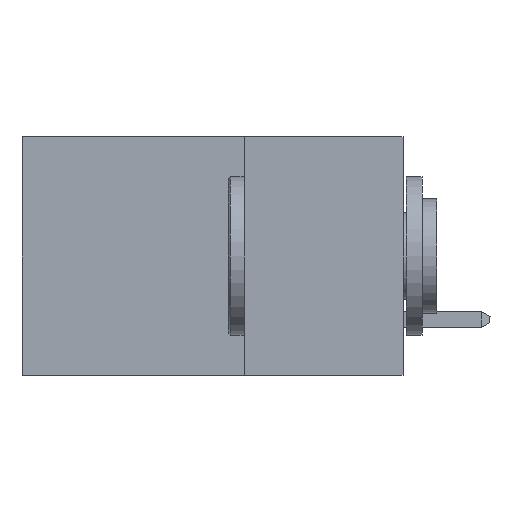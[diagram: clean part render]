
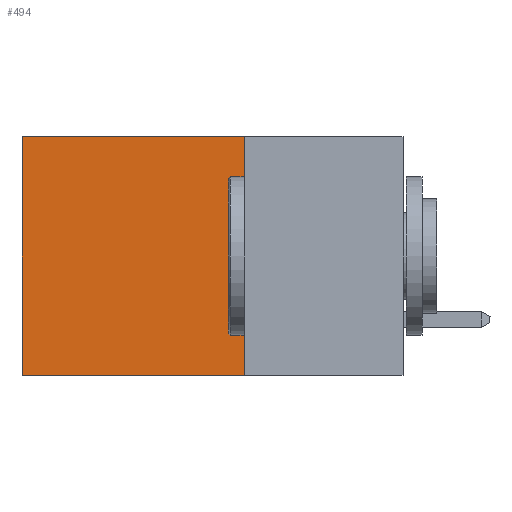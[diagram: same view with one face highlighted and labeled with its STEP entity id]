
A CAD part, left-side view. The second image highlights one B-rep face of the part: STEP entity #494.
In plain terms, the highlighted planar face has unit normal (-1, 0, 0).
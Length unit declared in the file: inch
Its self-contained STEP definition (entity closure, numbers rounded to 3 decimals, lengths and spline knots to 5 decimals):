
#149 = DIRECTION ( 'NONE',  ( 0., 0., -1. ) ) ;
#494 = ADVANCED_FACE ( 'NONE', ( #10853 ), #8749, .F. ) ;
#1987 = VECTOR ( 'NONE', #149, 39.37008 ) ;
#2050 = CARTESIAN_POINT ( 'NONE',  ( 0.2875, 0.25, 0. ) ) ;
#2059 = EDGE_LOOP ( 'NONE', ( #10766, #9060, #9444, #9440 ) ) ;
#3561 = EDGE_CURVE ( 'NONE', #10352, #12899, #7791, .T. ) ;
#3841 = EDGE_CURVE ( 'NONE', #8737, #8558, #11770, .T. ) ;
#4188 = CARTESIAN_POINT ( 'NONE',  ( 0.2875, 0.6, 0. ) ) ;
#4707 = CARTESIAN_POINT ( 'NONE',  ( 0.2875, 0.6, -0.375 ) ) ;
#5190 = VECTOR ( 'NONE', #9652, 39.37008 ) ;
#5316 = LINE ( 'NONE', #12598, #5190 ) ;
#5475 = CARTESIAN_POINT ( 'NONE',  ( 0.2875, 0.25, -0.375 ) ) ;
#6815 = DIRECTION ( 'NONE',  ( 0., 0., -1. ) ) ;
#7076 = CARTESIAN_POINT ( 'NONE',  ( 0.2875, 0.25, -0.375 ) ) ;
#7382 = AXIS2_PLACEMENT_3D ( 'NONE', #5475, #9733, #9868 ) ;
#7791 = LINE ( 'NONE', #4707, #10451 ) ;
#8365 = EDGE_CURVE ( 'NONE', #8558, #12899, #8839, .T. ) ;
#8407 = CARTESIAN_POINT ( 'NONE',  ( 0.2875, 0.25, -0.375 ) ) ;
#8558 = VERTEX_POINT ( 'NONE', #7076 ) ;
#8737 = VERTEX_POINT ( 'NONE', #2050 ) ;
#8749 = PLANE ( 'NONE',  #7382 ) ;
#8839 = LINE ( 'NONE', #12134, #9119 ) ;
#9060 = ORIENTED_EDGE ( 'NONE', *, *, #8365, .F. ) ;
#9119 = VECTOR ( 'NONE', #12199, 39.37008 ) ;
#9440 = ORIENTED_EDGE ( 'NONE', *, *, #12451, .T. ) ;
#9444 = ORIENTED_EDGE ( 'NONE', *, *, #3841, .F. ) ;
#9652 = DIRECTION ( 'NONE',  ( 0., 1., 0. ) ) ;
#9733 = DIRECTION ( 'NONE',  ( 1., 0., 0. ) ) ;
#9868 = DIRECTION ( 'NONE',  ( 0., 0., -1. ) ) ;
#10352 = VERTEX_POINT ( 'NONE', #4188 ) ;
#10451 = VECTOR ( 'NONE', #6815, 39.37008 ) ;
#10766 = ORIENTED_EDGE ( 'NONE', *, *, #3561, .T. ) ;
#10853 = FACE_OUTER_BOUND ( 'NONE', #2059, .T. ) ;
#10874 = CARTESIAN_POINT ( 'NONE',  ( 0.2875, 0.6, -0.375 ) ) ;
#11770 = LINE ( 'NONE', #8407, #1987 ) ;
#12134 = CARTESIAN_POINT ( 'NONE',  ( 0.2875, 0.25, -0.375 ) ) ;
#12199 = DIRECTION ( 'NONE',  ( 0., 1., 0. ) ) ;
#12451 = EDGE_CURVE ( 'NONE', #8737, #10352, #5316, .T. ) ;
#12598 = CARTESIAN_POINT ( 'NONE',  ( 0.2875, 0.25, 0. ) ) ;
#12899 = VERTEX_POINT ( 'NONE', #10874 ) ;
